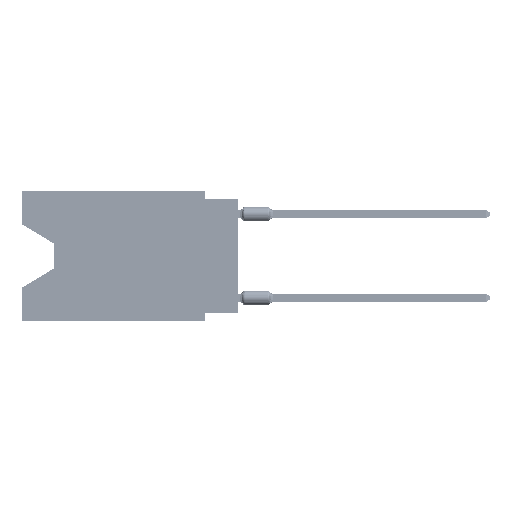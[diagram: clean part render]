
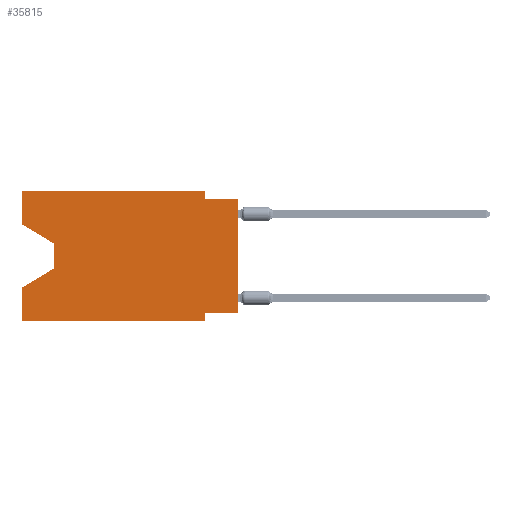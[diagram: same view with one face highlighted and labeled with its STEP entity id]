
A CAD part, left-side view. The second image highlights one B-rep face of the part: STEP entity #35815.
In plain terms, the highlighted planar face has unit normal (-1, 0, 0).
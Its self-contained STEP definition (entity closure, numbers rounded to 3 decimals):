
#300 = DIRECTION ( 'NONE',  ( 0., 0., -1. ) ) ;
#1411 = CARTESIAN_POINT ( 'NONE',  ( 0., 16.383, 0. ) ) ;
#1737 = CARTESIAN_POINT ( 'NONE',  ( 0., 0., -9.271 ) ) ;
#1883 = DIRECTION ( 'NONE',  ( 0., -1., 0. ) ) ;
#2119 = EDGE_CURVE ( 'NONE', #18832, #32674, #60295, .T. ) ;
#2915 = CARTESIAN_POINT ( 'NONE',  ( 0., 2.54, -0.635 ) ) ;
#3404 = DIRECTION ( 'NONE',  ( 0., 0.855, -0.519 ) ) ;
#3836 = VECTOR ( 'NONE', #3404, 1000. ) ;
#7489 = CARTESIAN_POINT ( 'NONE',  ( 0., 16.383, -9.906 ) ) ;
#7836 = PLANE ( 'NONE',  #9680 ) ;
#9233 = LINE ( 'NONE', #61391, #21363 ) ;
#9584 = VERTEX_POINT ( 'NONE', #50182 ) ;
#9680 = AXIS2_PLACEMENT_3D ( 'NONE', #1411, #41594, #48403 ) ;
#9809 = LINE ( 'NONE', #22221, #3836 ) ;
#10170 = CARTESIAN_POINT ( 'NONE',  ( 0., 0., -0.635 ) ) ;
#10279 = VECTOR ( 'NONE', #300, 1000. ) ;
#10566 = ORIENTED_EDGE ( 'NONE', *, *, #24842, .F. ) ;
#12303 = VECTOR ( 'NONE', #47755, 1000. ) ;
#12529 = CARTESIAN_POINT ( 'NONE',  ( 0., 2.54, -9.906 ) ) ;
#12955 = CARTESIAN_POINT ( 'NONE',  ( 0., 16.383, -2.546 ) ) ;
#13345 = EDGE_CURVE ( 'NONE', #34077, #19717, #14860, .T. ) ;
#13389 = DIRECTION ( 'NONE',  ( 0., -0.855, -0.519 ) ) ;
#14860 = LINE ( 'NONE', #71826, #12303 ) ;
#15282 = CARTESIAN_POINT ( 'NONE',  ( 0., 16.383, -2.546 ) ) ;
#15505 = FACE_OUTER_BOUND ( 'NONE', #45135, .T. ) ;
#16384 = ORIENTED_EDGE ( 'NONE', *, *, #67433, .T. ) ;
#16465 = VERTEX_POINT ( 'NONE', #68717 ) ;
#16507 = VECTOR ( 'NONE', #71869, 1000. ) ;
#17955 = ORIENTED_EDGE ( 'NONE', *, *, #76602, .F. ) ;
#18584 = ORIENTED_EDGE ( 'NONE', *, *, #2119, .F. ) ;
#18805 = VERTEX_POINT ( 'NONE', #2915 ) ;
#18832 = VERTEX_POINT ( 'NONE', #68296 ) ;
#18939 = ORIENTED_EDGE ( 'NONE', *, *, #57272, .T. ) ;
#19309 = VECTOR ( 'NONE', #27829, 1000. ) ;
#19717 = VERTEX_POINT ( 'NONE', #81332 ) ;
#19954 = VERTEX_POINT ( 'NONE', #10170 ) ;
#19958 = CARTESIAN_POINT ( 'NONE',  ( 0., 2.54, -9.906 ) ) ;
#20048 = CARTESIAN_POINT ( 'NONE',  ( 0., 13.97, -4.013 ) ) ;
#21363 = VECTOR ( 'NONE', #29762, 1000. ) ;
#21961 = LINE ( 'NONE', #48020, #73277 ) ;
#22221 = CARTESIAN_POINT ( 'NONE',  ( 0., 13.97, -5.893 ) ) ;
#22253 = EDGE_CURVE ( 'NONE', #9584, #18805, #81930, .T. ) ;
#22844 = EDGE_CURVE ( 'NONE', #76317, #16465, #45454, .T. ) ;
#24139 = VERTEX_POINT ( 'NONE', #33936 ) ;
#24315 = CARTESIAN_POINT ( 'NONE',  ( 0., 16.383, -9.906 ) ) ;
#24454 = VECTOR ( 'NONE', #53780, 1000. ) ;
#24842 = EDGE_CURVE ( 'NONE', #32674, #44714, #39207, .T. ) ;
#26748 = VECTOR ( 'NONE', #62693, 1000. ) ;
#27428 = ORIENTED_EDGE ( 'NONE', *, *, #82319, .T. ) ;
#27829 = DIRECTION ( 'NONE',  ( 0., 1., 0. ) ) ;
#29762 = DIRECTION ( 'NONE',  ( 0., 0., 1. ) ) ;
#30232 = CARTESIAN_POINT ( 'NONE',  ( 0., 2.54, -9.271 ) ) ;
#30700 = VECTOR ( 'NONE', #63128, 1000. ) ;
#32147 = EDGE_CURVE ( 'NONE', #24139, #19717, #9809, .T. ) ;
#32674 = VERTEX_POINT ( 'NONE', #30232 ) ;
#33936 = CARTESIAN_POINT ( 'NONE',  ( 0., 13.97, -5.893 ) ) ;
#34077 = VERTEX_POINT ( 'NONE', #7489 ) ;
#35815 = ADVANCED_FACE ( 'NONE', ( #15505 ), #7836, .F. ) ;
#37547 = ORIENTED_EDGE ( 'NONE', *, *, #32147, .T. ) ;
#38317 = LINE ( 'NONE', #57128, #26748 ) ;
#39207 = LINE ( 'NONE', #19958, #10279 ) ;
#39316 = ORIENTED_EDGE ( 'NONE', *, *, #13345, .F. ) ;
#41594 = DIRECTION ( 'NONE',  ( 1., 0., 0. ) ) ;
#44714 = VERTEX_POINT ( 'NONE', #12529 ) ;
#45135 = EDGE_LOOP ( 'NONE', ( #72371, #16384, #37547, #39316, #18939, #10566, #18584, #27428, #57468, #80777, #52118, #17955 ) ) ;
#45454 = LINE ( 'NONE', #12955, #49816 ) ;
#45789 = CARTESIAN_POINT ( 'NONE',  ( 0., 0., -0.635 ) ) ;
#47755 = DIRECTION ( 'NONE',  ( 0., 0., 1. ) ) ;
#48020 = CARTESIAN_POINT ( 'NONE',  ( 0., 16.383, 0. ) ) ;
#48403 = DIRECTION ( 'NONE',  ( 0., 0., -1. ) ) ;
#49816 = VECTOR ( 'NONE', #13389, 1000. ) ;
#50182 = CARTESIAN_POINT ( 'NONE',  ( 0., 2.54, 0. ) ) ;
#52118 = ORIENTED_EDGE ( 'NONE', *, *, #82811, .F. ) ;
#53780 = DIRECTION ( 'NONE',  ( 0., 0., -1. ) ) ;
#57128 = CARTESIAN_POINT ( 'NONE',  ( 0., 16.383, 0. ) ) ;
#57272 = EDGE_CURVE ( 'NONE', #34077, #44714, #81276, .T. ) ;
#57468 = ORIENTED_EDGE ( 'NONE', *, *, #69188, .F. ) ;
#57641 = VECTOR ( 'NONE', #80856, 1000. ) ;
#59470 = LINE ( 'NONE', #45789, #16507 ) ;
#60206 = LINE ( 'NONE', #20048, #24454 ) ;
#60295 = LINE ( 'NONE', #1737, #19309 ) ;
#61391 = CARTESIAN_POINT ( 'NONE',  ( 0., 0., 0. ) ) ;
#62693 = DIRECTION ( 'NONE',  ( 0., 0., 1. ) ) ;
#63128 = DIRECTION ( 'NONE',  ( 0., 0., -1. ) ) ;
#67433 = EDGE_CURVE ( 'NONE', #16465, #24139, #60206, .T. ) ;
#68296 = CARTESIAN_POINT ( 'NONE',  ( 0., 0., -9.271 ) ) ;
#68717 = CARTESIAN_POINT ( 'NONE',  ( 0., 13.97, -4.013 ) ) ;
#69188 = EDGE_CURVE ( 'NONE', #18805, #19954, #59470, .T. ) ;
#70489 = VERTEX_POINT ( 'NONE', #78712 ) ;
#71826 = CARTESIAN_POINT ( 'NONE',  ( 0., 16.383, 0. ) ) ;
#71869 = DIRECTION ( 'NONE',  ( 0., -1., 0. ) ) ;
#72371 = ORIENTED_EDGE ( 'NONE', *, *, #22844, .T. ) ;
#73277 = VECTOR ( 'NONE', #1883, 1000. ) ;
#76317 = VERTEX_POINT ( 'NONE', #15282 ) ;
#76602 = EDGE_CURVE ( 'NONE', #76317, #70489, #38317, .T. ) ;
#78712 = CARTESIAN_POINT ( 'NONE',  ( 0., 16.383, 0. ) ) ;
#80777 = ORIENTED_EDGE ( 'NONE', *, *, #22253, .F. ) ;
#80856 = DIRECTION ( 'NONE',  ( 0., -1., 0. ) ) ;
#81276 = LINE ( 'NONE', #24315, #57641 ) ;
#81332 = CARTESIAN_POINT ( 'NONE',  ( 0., 16.383, -7.36 ) ) ;
#81930 = LINE ( 'NONE', #82335, #30700 ) ;
#82319 = EDGE_CURVE ( 'NONE', #18832, #19954, #9233, .T. ) ;
#82335 = CARTESIAN_POINT ( 'NONE',  ( 0., 2.54, 0. ) ) ;
#82811 = EDGE_CURVE ( 'NONE', #70489, #9584, #21961, .T. ) ;
